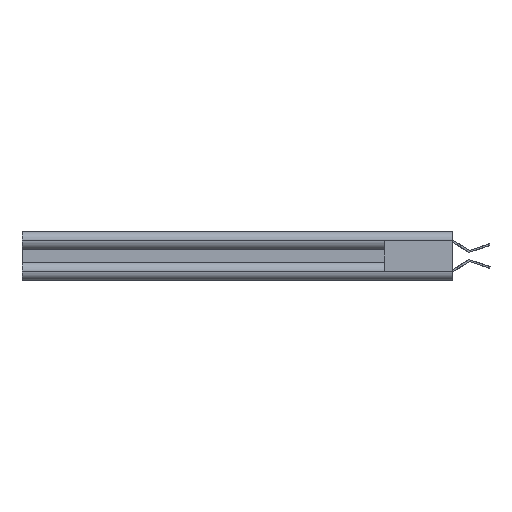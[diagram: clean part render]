
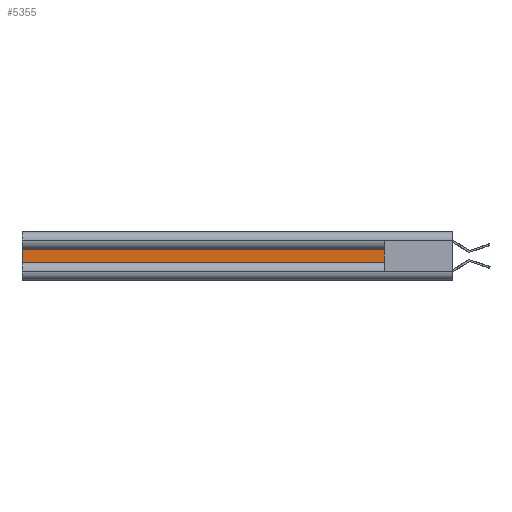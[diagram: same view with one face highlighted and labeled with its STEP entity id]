
A CAD part, left-side view. The second image highlights one B-rep face of the part: STEP entity #5355.
In plain terms, the highlighted planar face has unit normal (-1, 0, 0).
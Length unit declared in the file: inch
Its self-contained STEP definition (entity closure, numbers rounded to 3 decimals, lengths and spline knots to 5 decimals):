
#906 = EDGE_LOOP ( 'NONE', ( #10161, #2488, #11201, #1034 ) ) ;
#1034 = ORIENTED_EDGE ( 'NONE', *, *, #11577, .F. ) ;
#1773 = DIRECTION ( 'NONE',  ( 0., 0., -1. ) ) ;
#2488 = ORIENTED_EDGE ( 'NONE', *, *, #12156, .T. ) ;
#3066 = DIRECTION ( 'NONE',  ( 0., 1., 0. ) ) ;
#3341 = LINE ( 'NONE', #10625, #16698 ) ;
#4106 = VERTEX_POINT ( 'NONE', #4711 ) ;
#4150 = EDGE_CURVE ( 'NONE', #20845, #6411, #8298, .T. ) ;
#4711 = CARTESIAN_POINT ( 'NONE',  ( 0.044, 3., -0.0465 ) ) ;
#4719 = CARTESIAN_POINT ( 'NONE',  ( 0.044, 0.473, -0.0465 ) ) ;
#5355 = ADVANCED_FACE ( 'NONE', ( #9618 ), #22004, .F. ) ;
#6254 = CARTESIAN_POINT ( 'NONE',  ( 0.044, 3., 0.0465 ) ) ;
#6411 = VERTEX_POINT ( 'NONE', #6254 ) ;
#6768 = DIRECTION ( 'NONE',  ( 1., 0., 0. ) ) ;
#7300 = CARTESIAN_POINT ( 'NONE',  ( 0.044, 0.473, 0.0465 ) ) ;
#8298 = LINE ( 'NONE', #15289, #16880 ) ;
#8976 = DIRECTION ( 'NONE',  ( 0., 0., -1. ) ) ;
#9618 = FACE_OUTER_BOUND ( 'NONE', #906, .T. ) ;
#9811 = VECTOR ( 'NONE', #12289, 39.37008 ) ;
#10161 = ORIENTED_EDGE ( 'NONE', *, *, #4150, .T. ) ;
#10625 = CARTESIAN_POINT ( 'NONE',  ( 0.044, 0.473, -0.0465 ) ) ;
#11201 = ORIENTED_EDGE ( 'NONE', *, *, #21971, .F. ) ;
#11577 = EDGE_CURVE ( 'NONE', #20845, #17723, #3341, .T. ) ;
#12052 = AXIS2_PLACEMENT_3D ( 'NONE', #13658, #6768, #18762 ) ;
#12156 = EDGE_CURVE ( 'NONE', #6411, #4106, #14530, .T. ) ;
#12289 = DIRECTION ( 'NONE',  ( 0., 1., 0. ) ) ;
#13658 = CARTESIAN_POINT ( 'NONE',  ( 0.044, 0.37012, -0.0465 ) ) ;
#13981 = CARTESIAN_POINT ( 'NONE',  ( 0.044, 3., -0.0465 ) ) ;
#14387 = LINE ( 'NONE', #20726, #9811 ) ;
#14530 = LINE ( 'NONE', #13981, #17975 ) ;
#15289 = CARTESIAN_POINT ( 'NONE',  ( 0.044, 0.37012, 0.0465 ) ) ;
#16698 = VECTOR ( 'NONE', #8976, 39.37008 ) ;
#16880 = VECTOR ( 'NONE', #3066, 39.37008 ) ;
#17723 = VERTEX_POINT ( 'NONE', #4719 ) ;
#17975 = VECTOR ( 'NONE', #1773, 39.37008 ) ;
#18762 = DIRECTION ( 'NONE',  ( 0., 0., -1. ) ) ;
#20726 = CARTESIAN_POINT ( 'NONE',  ( 0.044, 0.37012, -0.0465 ) ) ;
#20845 = VERTEX_POINT ( 'NONE', #7300 ) ;
#21971 = EDGE_CURVE ( 'NONE', #17723, #4106, #14387, .T. ) ;
#22004 = PLANE ( 'NONE',  #12052 ) ;
